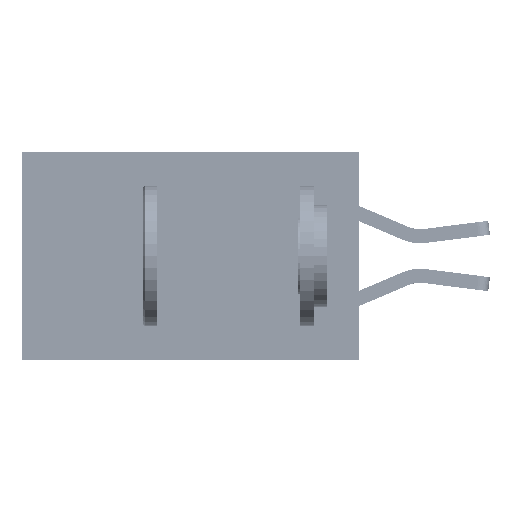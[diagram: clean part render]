
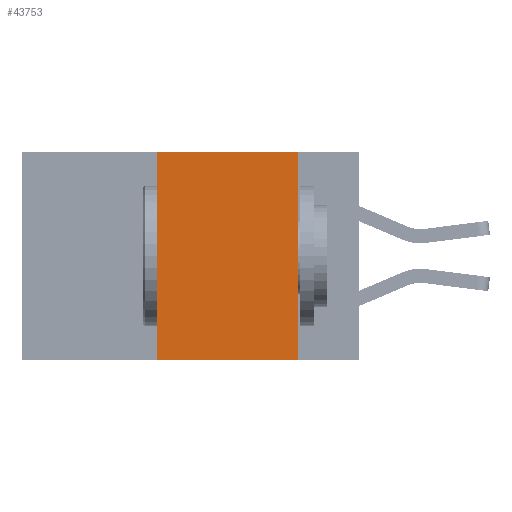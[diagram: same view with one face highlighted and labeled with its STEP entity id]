
A CAD part, left-side view. The second image highlights one B-rep face of the part: STEP entity #43753.
In plain terms, the highlighted planar face has unit normal (-1, 0, 0).
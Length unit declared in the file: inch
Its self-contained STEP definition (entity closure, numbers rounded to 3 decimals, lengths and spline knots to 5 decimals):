
#1307 = EDGE_CURVE ( 'NONE', #5431, #41385, #14655, .T. ) ;
#2025 = LINE ( 'NONE', #31681, #3872 ) ;
#2077 = EDGE_CURVE ( 'NONE', #22419, #5431, #50281, .T. ) ;
#2788 = CARTESIAN_POINT ( 'NONE',  ( 0., 0.6, 0. ) ) ;
#2867 = PLANE ( 'NONE',  #30213 ) ;
#3452 = VECTOR ( 'NONE', #16071, 39.37008 ) ;
#3872 = VECTOR ( 'NONE', #12033, 39.37008 ) ;
#3898 = EDGE_CURVE ( 'NONE', #41385, #33332, #2025, .T. ) ;
#5431 = VERTEX_POINT ( 'NONE', #22547 ) ;
#6222 = DIRECTION ( 'NONE',  ( 0., -1., 0. ) ) ;
#9112 = EDGE_LOOP ( 'NONE', ( #19387, #50847, #39273, #49395 ) ) ;
#9854 = VECTOR ( 'NONE', #22885, 39.37008 ) ;
#12033 = DIRECTION ( 'NONE',  ( 0., 0., -1. ) ) ;
#14655 = LINE ( 'NONE', #2788, #34372 ) ;
#16071 = DIRECTION ( 'NONE',  ( 0., 0., 1. ) ) ;
#17476 = FACE_OUTER_BOUND ( 'NONE', #9112, .T. ) ;
#19387 = ORIENTED_EDGE ( 'NONE', *, *, #3898, .F. ) ;
#21552 = LINE ( 'NONE', #38549, #9854 ) ;
#22419 = VERTEX_POINT ( 'NONE', #40238 ) ;
#22547 = CARTESIAN_POINT ( 'NONE',  ( 0., 0.36, 0. ) ) ;
#22885 = DIRECTION ( 'NONE',  ( 0., -1., 0. ) ) ;
#24924 = CARTESIAN_POINT ( 'NONE',  ( 0., 0.11, -0.37 ) ) ;
#26774 = DIRECTION ( 'NONE',  ( 0., 0., -1. ) ) ;
#27755 = CARTESIAN_POINT ( 'NONE',  ( 0., 0.36, 0. ) ) ;
#30213 = AXIS2_PLACEMENT_3D ( 'NONE', #50381, #34375, #26774 ) ;
#31681 = CARTESIAN_POINT ( 'NONE',  ( 0., 0.11, 0. ) ) ;
#33194 = CARTESIAN_POINT ( 'NONE',  ( 0., 0.11, 0. ) ) ;
#33332 = VERTEX_POINT ( 'NONE', #24924 ) ;
#34372 = VECTOR ( 'NONE', #6222, 39.37008 ) ;
#34375 = DIRECTION ( 'NONE',  ( 1., 0., 0. ) ) ;
#38549 = CARTESIAN_POINT ( 'NONE',  ( 0., 0.6, -0.37 ) ) ;
#39273 = ORIENTED_EDGE ( 'NONE', *, *, #2077, .F. ) ;
#40238 = CARTESIAN_POINT ( 'NONE',  ( 0., 0.36, -0.37 ) ) ;
#41385 = VERTEX_POINT ( 'NONE', #33194 ) ;
#43753 = ADVANCED_FACE ( 'NONE', ( #17476 ), #2867, .F. ) ;
#49159 = EDGE_CURVE ( 'NONE', #22419, #33332, #21552, .T. ) ;
#49395 = ORIENTED_EDGE ( 'NONE', *, *, #49159, .T. ) ;
#50281 = LINE ( 'NONE', #27755, #3452 ) ;
#50381 = CARTESIAN_POINT ( 'NONE',  ( 0., 0.6, 0. ) ) ;
#50847 = ORIENTED_EDGE ( 'NONE', *, *, #1307, .F. ) ;
